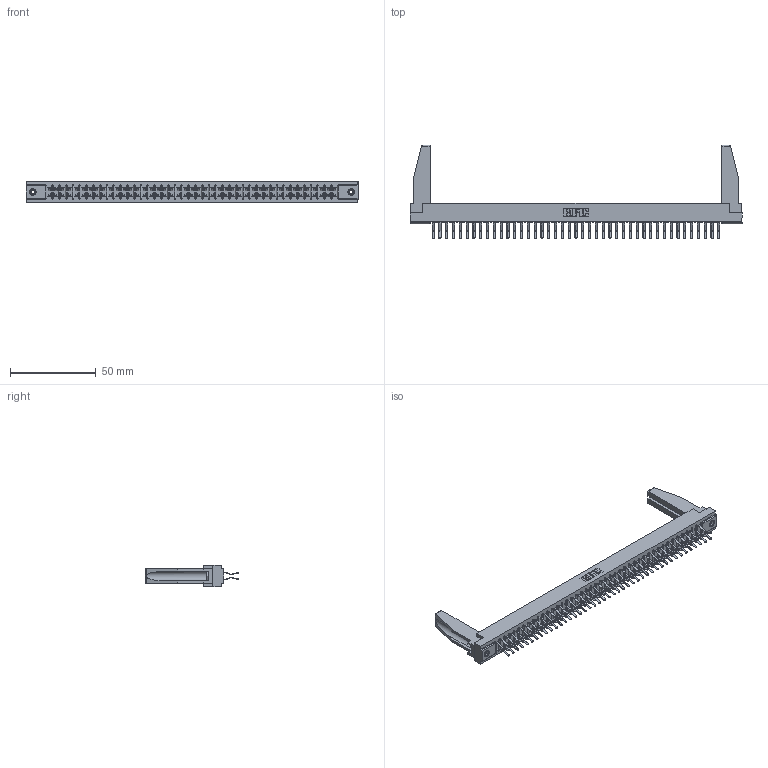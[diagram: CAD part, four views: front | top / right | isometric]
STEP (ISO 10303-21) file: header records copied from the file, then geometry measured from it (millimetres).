
FILE_DESCRIPTION (( 'STEP AP203' ), '1' );
FILE_NAME ('307-086-460-278.STEP', '2020-10-01T15:03:23', ( '' ), ( '' ), 'SwSTEP 2.0', 'SolidWorks 2020', '' );
FILE_SCHEMA (( 'CONFIG_CONTROL_DESIGN' ));
Length unit declared in the file: inch
Products named in the file (5): 307-086-460-278; 307-220-078; 345-250-001_345-250-001-102; 307 Part_.156 Dia Mounting Holes; 307-290-001_560
Assembly tree (91 placements, depth 2):
  307-086-460-278
    307 Part_.156 Dia Mounting Holes
    307-290-001_560  x86
    307-220-078  x2
    345-250-001_345-250-001-102  x2
Bounding box: 193.4 x 54.43 x 12.7 mm (x, y, z)
Volume: 24673 mm3; surface area: 29726.5 mm2
Topology: 91 solids, 91 shells, 4592 faces, 12865 edges, 8334 vertices
Faces by surface type: plane 2992, cylinder 1496, sphere 88, cone 12, torus 4
Entity records: 40659 total; most frequent: CARTESIAN_POINT 6661, ORIENTED_EDGE 6560, DIRECTION 6478, EDGE_CURVE 3280, LINE 2520, VECTOR 2520, VERTEX_POINT 2120, AXIS2_PLACEMENT_3D 1979
